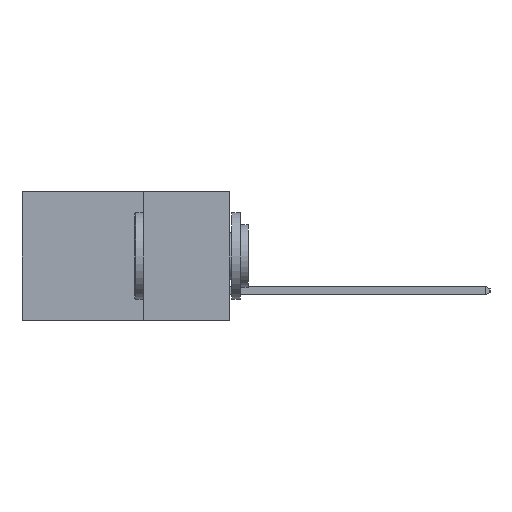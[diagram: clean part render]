
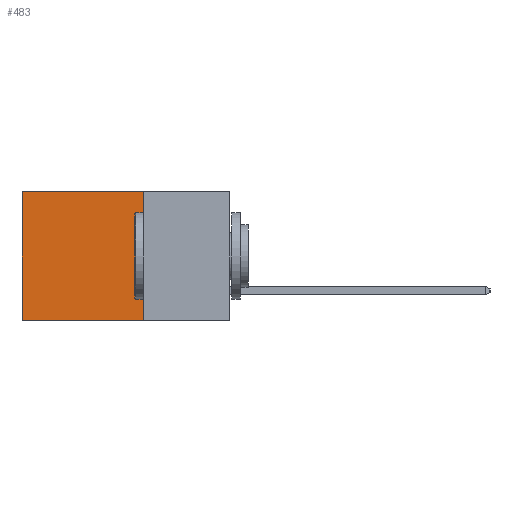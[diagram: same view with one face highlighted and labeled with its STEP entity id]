
A CAD part, left-side view. The second image highlights one B-rep face of the part: STEP entity #483.
In plain terms, the highlighted planar face has unit normal (-1, 0, 0).
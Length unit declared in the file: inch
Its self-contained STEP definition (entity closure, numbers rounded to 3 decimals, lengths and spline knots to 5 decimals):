
#261 = CARTESIAN_POINT ( 'NONE',  ( 0.2615, 0.6, -0.37 ) ) ;
#293 = VECTOR ( 'NONE', #8702, 39.37008 ) ;
#483 = ADVANCED_FACE ( 'NONE', ( #9302 ), #1999, .F. ) ;
#733 = DIRECTION ( 'NONE',  ( 0., 1., 0. ) ) ;
#1234 = DIRECTION ( 'NONE',  ( 0., 1., 0. ) ) ;
#1999 = PLANE ( 'NONE',  #10431 ) ;
#2142 = LINE ( 'NONE', #4744, #5432 ) ;
#2576 = LINE ( 'NONE', #9948, #8383 ) ;
#2596 = EDGE_LOOP ( 'NONE', ( #3417, #3482, #3599, #3743 ) ) ;
#3249 = DIRECTION ( 'NONE',  ( 0., 0., -1. ) ) ;
#3261 = EDGE_CURVE ( 'NONE', #12908, #11006, #2142, .T. ) ;
#3417 = ORIENTED_EDGE ( 'NONE', *, *, #10532, .T. ) ;
#3482 = ORIENTED_EDGE ( 'NONE', *, *, #3261, .F. ) ;
#3599 = ORIENTED_EDGE ( 'NONE', *, *, #15286, .F. ) ;
#3743 = ORIENTED_EDGE ( 'NONE', *, *, #9454, .T. ) ;
#4696 = VERTEX_POINT ( 'NONE', #10020 ) ;
#4744 = CARTESIAN_POINT ( 'NONE',  ( 0.2615, 0.25, -0.37 ) ) ;
#5432 = VECTOR ( 'NONE', #733, 39.37008 ) ;
#6567 = DIRECTION ( 'NONE',  ( 0., 0., -1. ) ) ;
#6725 = DIRECTION ( 'NONE',  ( 1., 0., 0. ) ) ;
#6805 = CARTESIAN_POINT ( 'NONE',  ( 0.2615, 0.25, -0.37 ) ) ;
#7466 = CARTESIAN_POINT ( 'NONE',  ( 0.2615, 0.25, -0.37 ) ) ;
#8383 = VECTOR ( 'NONE', #1234, 39.37008 ) ;
#8702 = DIRECTION ( 'NONE',  ( 0., 0., -1. ) ) ;
#9302 = FACE_OUTER_BOUND ( 'NONE', #2596, .T. ) ;
#9454 = EDGE_CURVE ( 'NONE', #4696, #9641, #2576, .T. ) ;
#9641 = VERTEX_POINT ( 'NONE', #14884 ) ;
#9896 = LINE ( 'NONE', #7466, #293 ) ;
#9948 = CARTESIAN_POINT ( 'NONE',  ( 0.2615, 0.25, 0. ) ) ;
#10020 = CARTESIAN_POINT ( 'NONE',  ( 0.2615, 0.25, 0. ) ) ;
#10122 = VECTOR ( 'NONE', #3249, 39.37008 ) ;
#10431 = AXIS2_PLACEMENT_3D ( 'NONE', #6805, #6725, #6567 ) ;
#10492 = LINE ( 'NONE', #15219, #10122 ) ;
#10532 = EDGE_CURVE ( 'NONE', #9641, #11006, #10492, .T. ) ;
#11006 = VERTEX_POINT ( 'NONE', #261 ) ;
#12908 = VERTEX_POINT ( 'NONE', #13534 ) ;
#13534 = CARTESIAN_POINT ( 'NONE',  ( 0.2615, 0.25, -0.37 ) ) ;
#14884 = CARTESIAN_POINT ( 'NONE',  ( 0.2615, 0.6, 0. ) ) ;
#15219 = CARTESIAN_POINT ( 'NONE',  ( 0.2615, 0.6, -0.37 ) ) ;
#15286 = EDGE_CURVE ( 'NONE', #4696, #12908, #9896, .T. ) ;
